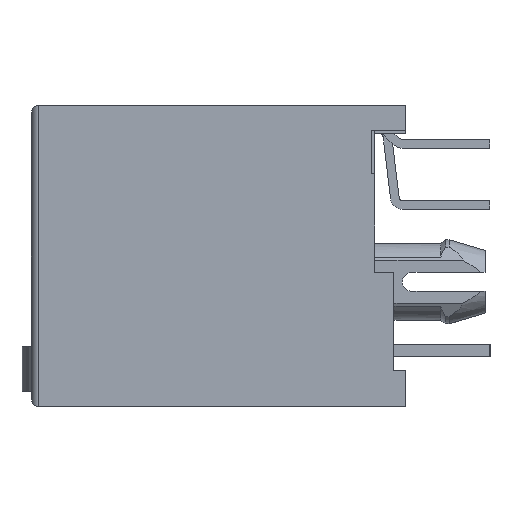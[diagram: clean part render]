
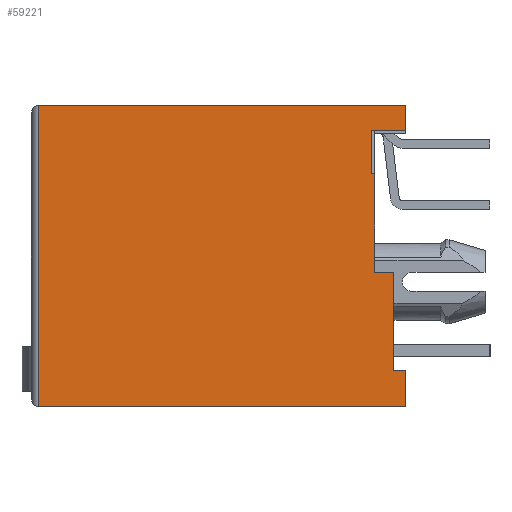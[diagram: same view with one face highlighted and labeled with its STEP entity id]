
A CAD part, left-side view. The second image highlights one B-rep face of the part: STEP entity #59221.
In plain terms, the highlighted planar face has unit normal (-1, 0, 0).
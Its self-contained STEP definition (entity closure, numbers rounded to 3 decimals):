
#590 = CARTESIAN_POINT ( 'NONE',  ( -31.5, -7.3, -4.75 ) ) ;
#620 = B_SPLINE_CURVE_WITH_KNOTS ( 'NONE', 3,
 ( #52142, #25514, #3705, #63039 ),
 .UNSPECIFIED., .F., .F.,
 ( 4, 4 ),
 ( 0., 1. ),
 .UNSPECIFIED. ) ;
#767 = B_SPLINE_CURVE_WITH_KNOTS ( 'NONE', 3,
 ( #16395, #5957, #49421, #16844 ),
 .UNSPECIFIED., .F., .F.,
 ( 4, 4 ),
 ( 0., 1. ),
 .UNSPECIFIED. ) ;
#913 = CARTESIAN_POINT ( 'NONE',  ( -31.5, -6.35, 4.05 ) ) ;
#1140 = CARTESIAN_POINT ( 'NONE',  ( -31.5, -6.35, 4.65 ) ) ;
#1591 = CARTESIAN_POINT ( 'NONE',  ( -31.5, -6.5, 3.45 ) ) ;
#1662 = B_SPLINE_CURVE_WITH_KNOTS ( 'NONE', 3,
 ( #36006, #8917, #52369, #19801 ),
 .UNSPECIFIED., .F., .F.,
 ( 4, 4 ),
 ( 0., 1. ),
 .UNSPECIFIED. ) ;
#1745 = CARTESIAN_POINT ( 'NONE',  ( -31.5, -7.033, -0.65 ) ) ;
#1964 = VERTEX_POINT ( 'NONE', #590 ) ;
#2229 = CARTESIAN_POINT ( 'NONE',  ( -31.5, -6.45, 3.45 ) ) ;
#2830 = EDGE_CURVE ( 'NONE', #15471, #60042, #1662, .T. ) ;
#3421 = VERTEX_POINT ( 'NONE', #19726 ) ;
#3705 = CARTESIAN_POINT ( 'NONE',  ( -31.5, 7.5, -2.067 ) ) ;
#3910 = VERTEX_POINT ( 'NONE', #25521 ) ;
#5957 = CARTESIAN_POINT ( 'NONE',  ( -31.5, -2.7, -6.25 ) ) ;
#6229 = EDGE_CURVE ( 'NONE', #3421, #62562, #31143, .T. ) ;
#7178 = CARTESIAN_POINT ( 'NONE',  ( -31.5, -7.3, -0.65 ) ) ;
#7254 = CARTESIAN_POINT ( 'NONE',  ( -31.5, -6.5, 2.083 ) ) ;
#8633 = ORIENTED_EDGE ( 'NONE', *, *, #2830, .F. ) ;
#8917 = CARTESIAN_POINT ( 'NONE',  ( -31.5, -7.317, 5.25 ) ) ;
#9220 = CARTESIAN_POINT ( 'NONE',  ( -31.5, -6.35, 5.25 ) ) ;
#9403 = FACE_OUTER_BOUND ( 'NONE', #37469, .T. ) ;
#10145 = B_SPLINE_CURVE_WITH_KNOTS ( 'NONE', 3,
 ( #67435, #51366, #52982, #31377 ),
 .UNSPECIFIED., .F., .F.,
 ( 4, 4 ),
 ( 0., 1. ),
 .UNSPECIFIED. ) ;
#10324 = EDGE_CURVE ( 'NONE', #32632, #54139, #620, .T. ) ;
#10331 = DIRECTION ( 'NONE',  ( 0., 0., 1. ) ) ;
#10388 = EDGE_CURVE ( 'NONE', #1964, #3910, #27101, .T. ) ;
#10834 = EDGE_CURVE ( 'NONE', #58844, #1964, #10145, .T. ) ;
#10978 = CARTESIAN_POINT ( 'NONE',  ( -31.5, -7.8, 5.6 ) ) ;
#11656 = CARTESIAN_POINT ( 'NONE',  ( -31.5, -7.8, 6.3 ) ) ;
#13862 = CARTESIAN_POINT ( 'NONE',  ( -31.5, -6.5, -0.65 ) ) ;
#14349 = B_SPLINE_CURVE_WITH_KNOTS ( 'NONE', 3,
 ( #53709, #38313, #10978, #42804 ),
 .UNSPECIFIED., .F., .F.,
 ( 4, 4 ),
 ( 0., 1. ),
 .UNSPECIFIED. ) ;
#15145 = ORIENTED_EDGE ( 'NONE', *, *, #29784, .T. ) ;
#15471 = VERTEX_POINT ( 'NONE', #39986 ) ;
#16395 = CARTESIAN_POINT ( 'NONE',  ( -31.5, -7.8, -6.25 ) ) ;
#16844 = CARTESIAN_POINT ( 'NONE',  ( -31.5, 7.5, -6.25 ) ) ;
#17353 = AXIS2_PLACEMENT_3D ( 'NONE', #22140, #64415, #10331 ) ;
#17605 = CARTESIAN_POINT ( 'NONE',  ( -31.5, -6.5, -0.65 ) ) ;
#18137 = ORIENTED_EDGE ( 'NONE', *, *, #6229, .F. ) ;
#18173 = CARTESIAN_POINT ( 'NONE',  ( -31.5, -7.3, -0.65 ) ) ;
#18887 = ORIENTED_EDGE ( 'NONE', *, *, #10324, .T. ) ;
#19077 = EDGE_CURVE ( 'NONE', #60042, #41759, #29190, .T. ) ;
#19726 = CARTESIAN_POINT ( 'NONE',  ( -31.5, -6.5, 3.45 ) ) ;
#19801 = CARTESIAN_POINT ( 'NONE',  ( -31.5, -6.35, 5.25 ) ) ;
#20018 = CARTESIAN_POINT ( 'NONE',  ( -31.5, -7.3, -4.75 ) ) ;
#22140 = CARTESIAN_POINT ( 'NONE',  ( -31.5, 7.806, -6.501 ) ) ;
#22163 = CARTESIAN_POINT ( 'NONE',  ( -31.5, -7.8, -5.75 ) ) ;
#22209 = CARTESIAN_POINT ( 'NONE',  ( -31.5, -6.35, 5.25 ) ) ;
#22276 = CARTESIAN_POINT ( 'NONE',  ( -31.5, -6.35, 3.45 ) ) ;
#23307 = CARTESIAN_POINT ( 'NONE',  ( -31.5, 7.5, -6.25 ) ) ;
#24662 = B_SPLINE_CURVE_WITH_KNOTS ( 'NONE', 3,
 ( #68917, #68685, #62817, #63050 ),
 .UNSPECIFIED., .F., .F.,
 ( 4, 4 ),
 ( 0., 1. ),
 .UNSPECIFIED. ) ;
#25514 = CARTESIAN_POINT ( 'NONE',  ( -31.5, 7.5, 2.117 ) ) ;
#25521 = CARTESIAN_POINT ( 'NONE',  ( -31.5, -7.8, -4.75 ) ) ;
#25893 = B_SPLINE_CURVE_WITH_KNOTS ( 'NONE', 3,
 ( #17605, #28309, #1745, #7178 ),
 .UNSPECIFIED., .F., .F.,
 ( 4, 4 ),
 ( 0., 1. ),
 .UNSPECIFIED. ) ;
#26971 = B_SPLINE_CURVE_WITH_KNOTS ( 'NONE', 3,
 ( #65378, #54726, #22163, #27881 ),
 .UNSPECIFIED., .F., .F.,
 ( 4, 4 ),
 ( 0., 1. ),
 .UNSPECIFIED. ) ;
#27101 = B_SPLINE_CURVE_WITH_KNOTS ( 'NONE', 3,
 ( #20018, #57083, #62569, #67990 ),
 .UNSPECIFIED., .F., .F.,
 ( 4, 4 ),
 ( 0., 1. ),
 .UNSPECIFIED. ) ;
#27881 = CARTESIAN_POINT ( 'NONE',  ( -31.5, -7.8, -6.25 ) ) ;
#28309 = CARTESIAN_POINT ( 'NONE',  ( -31.5, -6.767, -0.65 ) ) ;
#29190 = B_SPLINE_CURVE_WITH_KNOTS ( 'NONE', 3,
 ( #22209, #1140, #913, #60913 ),
 .UNSPECIFIED., .F., .F.,
 ( 4, 4 ),
 ( 0., 1. ),
 .UNSPECIFIED. ) ;
#29567 = CARTESIAN_POINT ( 'NONE',  ( -31.5, -6.5, 0.717 ) ) ;
#29784 = EDGE_CURVE ( 'NONE', #47733, #32632, #24662, .T. ) ;
#30026 = CARTESIAN_POINT ( 'NONE',  ( -31.5, -6.5, -0.65 ) ) ;
#30132 = EDGE_CURVE ( 'NONE', #41759, #3421, #64699, .T. ) ;
#31089 = EDGE_CURVE ( 'NONE', #57096, #54139, #767, .T. ) ;
#31143 = B_SPLINE_CURVE_WITH_KNOTS ( 'NONE', 3,
 ( #1591, #7254, #29567, #30026 ),
 .UNSPECIFIED., .F., .F.,
 ( 4, 4 ),
 ( 0., 1. ),
 .UNSPECIFIED. ) ;
#31377 = CARTESIAN_POINT ( 'NONE',  ( -31.5, -7.3, -4.75 ) ) ;
#32199 = PLANE ( 'NONE',  #17353 ) ;
#32632 = VERTEX_POINT ( 'NONE', #34982 ) ;
#32967 = ORIENTED_EDGE ( 'NONE', *, *, #56160, .F. ) ;
#32988 = CARTESIAN_POINT ( 'NONE',  ( -31.5, -7.8, -6.25 ) ) ;
#34760 = ORIENTED_EDGE ( 'NONE', *, *, #64657, .F. ) ;
#34982 = CARTESIAN_POINT ( 'NONE',  ( -31.5, 7.5, 6.3 ) ) ;
#36006 = CARTESIAN_POINT ( 'NONE',  ( -31.5, -7.8, 5.25 ) ) ;
#37469 = EDGE_LOOP ( 'NONE', ( #32967, #47775, #67699, #34760, #18137, #47312, #56531, #8633, #60655, #15145, #18887, #64809 ) ) ;
#38313 = CARTESIAN_POINT ( 'NONE',  ( -31.5, -7.8, 5.95 ) ) ;
#38835 = CARTESIAN_POINT ( 'NONE',  ( -31.5, -6.4, 3.45 ) ) ;
#39986 = CARTESIAN_POINT ( 'NONE',  ( -31.5, -7.8, 5.25 ) ) ;
#41759 = VERTEX_POINT ( 'NONE', #22276 ) ;
#42804 = CARTESIAN_POINT ( 'NONE',  ( -31.5, -7.8, 5.25 ) ) ;
#43805 = CARTESIAN_POINT ( 'NONE',  ( -31.5, -6.35, 3.45 ) ) ;
#47312 = ORIENTED_EDGE ( 'NONE', *, *, #30132, .F. ) ;
#47733 = VERTEX_POINT ( 'NONE', #11656 ) ;
#47775 = ORIENTED_EDGE ( 'NONE', *, *, #10388, .F. ) ;
#49421 = CARTESIAN_POINT ( 'NONE',  ( -31.5, 2.4, -6.25 ) ) ;
#51366 = CARTESIAN_POINT ( 'NONE',  ( -31.5, -7.3, -2.017 ) ) ;
#52142 = CARTESIAN_POINT ( 'NONE',  ( -31.5, 7.5, 6.3 ) ) ;
#52369 = CARTESIAN_POINT ( 'NONE',  ( -31.5, -6.833, 5.25 ) ) ;
#52982 = CARTESIAN_POINT ( 'NONE',  ( -31.5, -7.3, -3.383 ) ) ;
#53709 = CARTESIAN_POINT ( 'NONE',  ( -31.5, -7.8, 6.3 ) ) ;
#54139 = VERTEX_POINT ( 'NONE', #23307 ) ;
#54726 = CARTESIAN_POINT ( 'NONE',  ( -31.5, -7.8, -5.25 ) ) ;
#56160 = EDGE_CURVE ( 'NONE', #3910, #57096, #26971, .T. ) ;
#56531 = ORIENTED_EDGE ( 'NONE', *, *, #19077, .F. ) ;
#56536 = EDGE_CURVE ( 'NONE', #47733, #15471, #14349, .T. ) ;
#57083 = CARTESIAN_POINT ( 'NONE',  ( -31.5, -7.467, -4.75 ) ) ;
#57096 = VERTEX_POINT ( 'NONE', #32988 ) ;
#58844 = VERTEX_POINT ( 'NONE', #18173 ) ;
#59221 = ADVANCED_FACE ( 'NONE', ( #9403 ), #32199, .F. ) ;
#60042 = VERTEX_POINT ( 'NONE', #9220 ) ;
#60655 = ORIENTED_EDGE ( 'NONE', *, *, #56536, .F. ) ;
#60913 = CARTESIAN_POINT ( 'NONE',  ( -31.5, -6.35, 3.45 ) ) ;
#62562 = VERTEX_POINT ( 'NONE', #13862 ) ;
#62569 = CARTESIAN_POINT ( 'NONE',  ( -31.5, -7.633, -4.75 ) ) ;
#62817 = CARTESIAN_POINT ( 'NONE',  ( -31.5, 2.4, 6.3 ) ) ;
#63039 = CARTESIAN_POINT ( 'NONE',  ( -31.5, 7.5, -6.25 ) ) ;
#63050 = CARTESIAN_POINT ( 'NONE',  ( -31.5, 7.5, 6.3 ) ) ;
#64415 = DIRECTION ( 'NONE',  ( 1., 0., 0. ) ) ;
#64657 = EDGE_CURVE ( 'NONE', #62562, #58844, #25893, .T. ) ;
#64699 = B_SPLINE_CURVE_WITH_KNOTS ( 'NONE', 3,
 ( #43805, #38835, #2229, #67219 ),
 .UNSPECIFIED., .F., .F.,
 ( 4, 4 ),
 ( 0., 1. ),
 .UNSPECIFIED. ) ;
#64809 = ORIENTED_EDGE ( 'NONE', *, *, #31089, .F. ) ;
#65378 = CARTESIAN_POINT ( 'NONE',  ( -31.5, -7.8, -4.75 ) ) ;
#67219 = CARTESIAN_POINT ( 'NONE',  ( -31.5, -6.5, 3.45 ) ) ;
#67435 = CARTESIAN_POINT ( 'NONE',  ( -31.5, -7.3, -0.65 ) ) ;
#67699 = ORIENTED_EDGE ( 'NONE', *, *, #10834, .F. ) ;
#67990 = CARTESIAN_POINT ( 'NONE',  ( -31.5, -7.8, -4.75 ) ) ;
#68685 = CARTESIAN_POINT ( 'NONE',  ( -31.5, -2.7, 6.3 ) ) ;
#68917 = CARTESIAN_POINT ( 'NONE',  ( -31.5, -7.8, 6.3 ) ) ;
